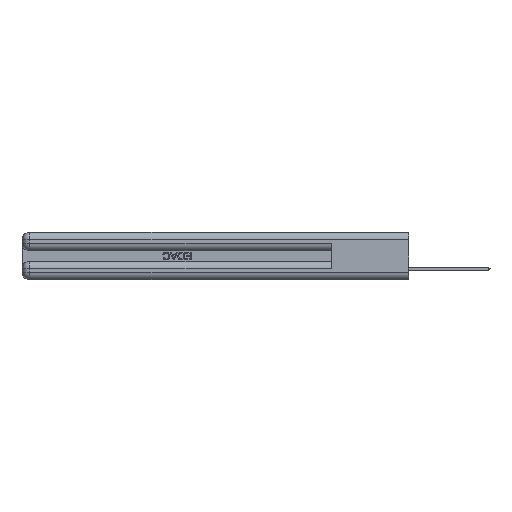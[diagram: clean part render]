
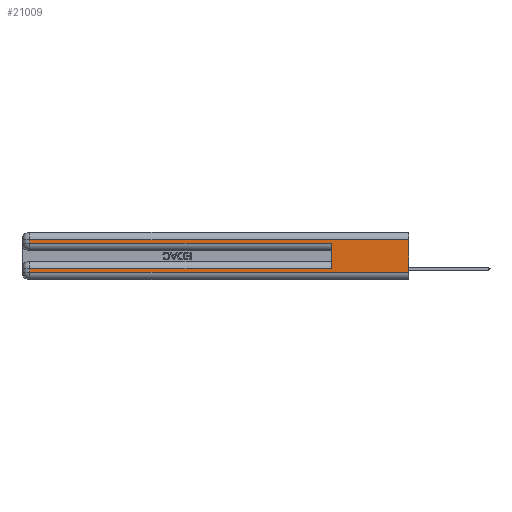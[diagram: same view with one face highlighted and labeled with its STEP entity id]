
A CAD part, left-side view. The second image highlights one B-rep face of the part: STEP entity #21009.
In plain terms, the highlighted planar face has unit normal (-1, 0, 0).
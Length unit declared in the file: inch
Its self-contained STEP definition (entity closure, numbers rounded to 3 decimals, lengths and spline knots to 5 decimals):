
#1635 = ORIENTED_EDGE ( 'NONE', *, *, #12677, .T. ) ;
#1768 = LINE ( 'NONE', #16402, #16007 ) ;
#3571 = LINE ( 'NONE', #14736, #10433 ) ;
#3647 = VERTEX_POINT ( 'NONE', #8716 ) ;
#3666 = ORIENTED_EDGE ( 'NONE', *, *, #33382, .T. ) ;
#5178 = LINE ( 'NONE', #36216, #33104 ) ;
#5716 = EDGE_CURVE ( 'NONE', #26190, #3647, #42643, .T. ) ;
#6882 = CARTESIAN_POINT ( 'NONE',  ( 0., 2.94, 0.31 ) ) ;
#6909 = CARTESIAN_POINT ( 'NONE',  ( 0., 0., 0.06 ) ) ;
#7112 = CARTESIAN_POINT ( 'NONE',  ( 0., 0.6, 0.285 ) ) ;
#8122 = CARTESIAN_POINT ( 'NONE',  ( 0., 0., 0.31 ) ) ;
#8533 = VECTOR ( 'NONE', #43507, 39.37008 ) ;
#8538 = ORIENTED_EDGE ( 'NONE', *, *, #41725, .T. ) ;
#8716 = CARTESIAN_POINT ( 'NONE',  ( 0., 2.94, 0.285 ) ) ;
#8921 = EDGE_CURVE ( 'NONE', #14382, #13442, #3571, .T. ) ;
#10391 = ORIENTED_EDGE ( 'NONE', *, *, #26881, .F. ) ;
#10433 = VECTOR ( 'NONE', #43952, 39.37008 ) ;
#12142 = VERTEX_POINT ( 'NONE', #7112 ) ;
#12677 = EDGE_CURVE ( 'NONE', #3647, #12142, #1768, .T. ) ;
#13442 = VERTEX_POINT ( 'NONE', #16396 ) ;
#14382 = VERTEX_POINT ( 'NONE', #24535 ) ;
#14736 = CARTESIAN_POINT ( 'NONE',  ( 0., 2.94, 0.37 ) ) ;
#15731 = VERTEX_POINT ( 'NONE', #35099 ) ;
#16007 = VECTOR ( 'NONE', #16238, 39.37008 ) ;
#16238 = DIRECTION ( 'NONE',  ( 0., -1., 0. ) ) ;
#16396 = CARTESIAN_POINT ( 'NONE',  ( 0., 2.94, 0.06 ) ) ;
#16402 = CARTESIAN_POINT ( 'NONE',  ( 0., 0., 0.285 ) ) ;
#16509 = VECTOR ( 'NONE', #26888, 39.37008 ) ;
#17773 = EDGE_LOOP ( 'NONE', ( #21847, #3666, #46613, #1635, #10391, #8538, #27302, #42577 ) ) ;
#17889 = VECTOR ( 'NONE', #21869, 39.37008 ) ;
#21009 = ADVANCED_FACE ( 'NONE', ( #28443 ), #46815, .F. ) ;
#21847 = ORIENTED_EDGE ( 'NONE', *, *, #41525, .F. ) ;
#21869 = DIRECTION ( 'NONE',  ( 0., -1., 0. ) ) ;
#24535 = CARTESIAN_POINT ( 'NONE',  ( 0., 2.94, 0.085 ) ) ;
#25653 = VERTEX_POINT ( 'NONE', #6909 ) ;
#26190 = VERTEX_POINT ( 'NONE', #6882 ) ;
#26472 = LINE ( 'NONE', #27310, #44721 ) ;
#26881 = EDGE_CURVE ( 'NONE', #15731, #12142, #26472, .T. ) ;
#26888 = DIRECTION ( 'NONE',  ( 0., 1., 0. ) ) ;
#27302 = ORIENTED_EDGE ( 'NONE', *, *, #8921, .T. ) ;
#27310 = CARTESIAN_POINT ( 'NONE',  ( 0., 0.6, 0.145 ) ) ;
#28318 = CARTESIAN_POINT ( 'NONE',  ( 0., 0., 0.37 ) ) ;
#28443 = FACE_OUTER_BOUND ( 'NONE', #17773, .T. ) ;
#30987 = VERTEX_POINT ( 'NONE', #8122 ) ;
#32434 = DIRECTION ( 'NONE',  ( 1., 0., 0. ) ) ;
#32552 = DIRECTION ( 'NONE',  ( 0., 0., -1. ) ) ;
#32691 = CARTESIAN_POINT ( 'NONE',  ( 0., 0., 0.06 ) ) ;
#33104 = VECTOR ( 'NONE', #35589, 39.37008 ) ;
#33382 = EDGE_CURVE ( 'NONE', #30987, #26190, #5178, .T. ) ;
#34764 = LINE ( 'NONE', #46680, #8533 ) ;
#35099 = CARTESIAN_POINT ( 'NONE',  ( 0., 0.6, 0.085 ) ) ;
#35589 = DIRECTION ( 'NONE',  ( 0., 1., 0. ) ) ;
#36216 = CARTESIAN_POINT ( 'NONE',  ( 0., 0., 0.31 ) ) ;
#39062 = DIRECTION ( 'NONE',  ( 0., 0., 1. ) ) ;
#39127 = AXIS2_PLACEMENT_3D ( 'NONE', #28318, #32434, #39596 ) ;
#39596 = DIRECTION ( 'NONE',  ( 0., 0., -1. ) ) ;
#39723 = CARTESIAN_POINT ( 'NONE',  ( 0., 2.94, 0.37 ) ) ;
#39833 = LINE ( 'NONE', #41055, #16509 ) ;
#41055 = CARTESIAN_POINT ( 'NONE',  ( 0., 0., 0.085 ) ) ;
#41525 = EDGE_CURVE ( 'NONE', #30987, #25653, #34764, .T. ) ;
#41725 = EDGE_CURVE ( 'NONE', #15731, #14382, #39833, .T. ) ;
#42577 = ORIENTED_EDGE ( 'NONE', *, *, #45176, .T. ) ;
#42643 = LINE ( 'NONE', #39723, #43207 ) ;
#43207 = VECTOR ( 'NONE', #32552, 39.37008 ) ;
#43507 = DIRECTION ( 'NONE',  ( 0., 0., -1. ) ) ;
#43952 = DIRECTION ( 'NONE',  ( 0., 0., -1. ) ) ;
#44139 = LINE ( 'NONE', #32691, #17889 ) ;
#44721 = VECTOR ( 'NONE', #39062, 39.37008 ) ;
#45176 = EDGE_CURVE ( 'NONE', #13442, #25653, #44139, .T. ) ;
#46613 = ORIENTED_EDGE ( 'NONE', *, *, #5716, .T. ) ;
#46680 = CARTESIAN_POINT ( 'NONE',  ( 0., 0., 0.37 ) ) ;
#46815 = PLANE ( 'NONE',  #39127 ) ;
